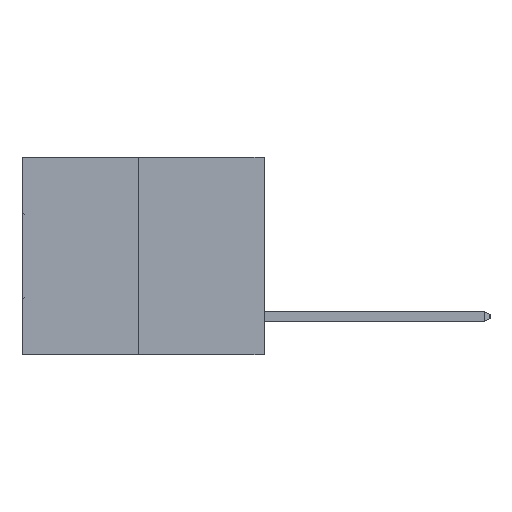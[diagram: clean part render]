
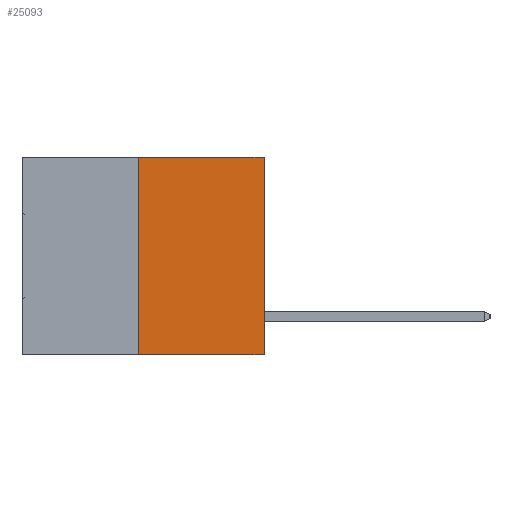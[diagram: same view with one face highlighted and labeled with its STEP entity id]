
A CAD part, left-side view. The second image highlights one B-rep face of the part: STEP entity #25093.
In plain terms, the highlighted planar face has unit normal (-1, 0, 0).
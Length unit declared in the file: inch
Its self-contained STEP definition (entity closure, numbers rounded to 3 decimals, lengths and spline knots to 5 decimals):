
#1457 = DIRECTION ( 'NONE',  ( 0., -1., 0. ) ) ;
#2105 = CARTESIAN_POINT ( 'NONE',  ( 0., 0.6, -0.49 ) ) ;
#3389 = VERTEX_POINT ( 'NONE', #10623 ) ;
#4869 = ORIENTED_EDGE ( 'NONE', *, *, #31299, .F. ) ;
#4993 = DIRECTION ( 'NONE',  ( 0., -1., 0. ) ) ;
#6207 = VERTEX_POINT ( 'NONE', #6440 ) ;
#6440 = CARTESIAN_POINT ( 'NONE',  ( 0., 0., 0. ) ) ;
#7290 = FACE_OUTER_BOUND ( 'NONE', #13647, .T. ) ;
#8166 = LINE ( 'NONE', #2105, #23605 ) ;
#10623 = CARTESIAN_POINT ( 'NONE',  ( 0., 0.312, -0.49 ) ) ;
#13493 = CARTESIAN_POINT ( 'NONE',  ( 0., 0.312, 0. ) ) ;
#13647 = EDGE_LOOP ( 'NONE', ( #29042, #16586, #27812, #4869 ) ) ;
#15043 = CARTESIAN_POINT ( 'NONE',  ( 0., 0.6, 0. ) ) ;
#15818 = VERTEX_POINT ( 'NONE', #24495 ) ;
#16586 = ORIENTED_EDGE ( 'NONE', *, *, #23310, .T. ) ;
#18619 = EDGE_CURVE ( 'NONE', #15818, #6207, #30948, .T. ) ;
#22586 = VECTOR ( 'NONE', #29607, 39.37008 ) ;
#23019 = DIRECTION ( 'NONE',  ( 0., 0., -1. ) ) ;
#23310 = EDGE_CURVE ( 'NONE', #3389, #15818, #8166, .T. ) ;
#23480 = VECTOR ( 'NONE', #1457, 39.37008 ) ;
#23605 = VECTOR ( 'NONE', #4993, 39.37008 ) ;
#24495 = CARTESIAN_POINT ( 'NONE',  ( 0., 0., -0.49 ) ) ;
#24505 = DIRECTION ( 'NONE',  ( 0., 0., 1. ) ) ;
#24741 = LINE ( 'NONE', #30783, #23480 ) ;
#25093 = ADVANCED_FACE ( 'NONE', ( #7290 ), #33636, .F. ) ;
#25708 = VECTOR ( 'NONE', #24505, 39.37008 ) ;
#25981 = VERTEX_POINT ( 'NONE', #13493 ) ;
#27812 = ORIENTED_EDGE ( 'NONE', *, *, #18619, .T. ) ;
#28488 = DIRECTION ( 'NONE',  ( 1., 0., 0. ) ) ;
#29042 = ORIENTED_EDGE ( 'NONE', *, *, #30913, .F. ) ;
#29607 = DIRECTION ( 'NONE',  ( 0., 0., 1. ) ) ;
#29882 = CARTESIAN_POINT ( 'NONE',  ( 0., 0.312, -0.49 ) ) ;
#30783 = CARTESIAN_POINT ( 'NONE',  ( 0., 0.6, 0. ) ) ;
#30913 = EDGE_CURVE ( 'NONE', #3389, #25981, #31180, .T. ) ;
#30948 = LINE ( 'NONE', #32191, #22586 ) ;
#31180 = LINE ( 'NONE', #29882, #25708 ) ;
#31299 = EDGE_CURVE ( 'NONE', #25981, #6207, #24741, .T. ) ;
#32191 = CARTESIAN_POINT ( 'NONE',  ( 0., 0., 0. ) ) ;
#33636 = PLANE ( 'NONE',  #34210 ) ;
#34210 = AXIS2_PLACEMENT_3D ( 'NONE', #15043, #28488, #23019 ) ;
